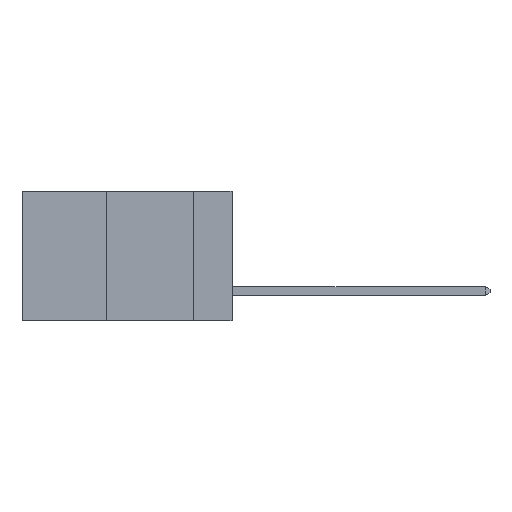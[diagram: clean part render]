
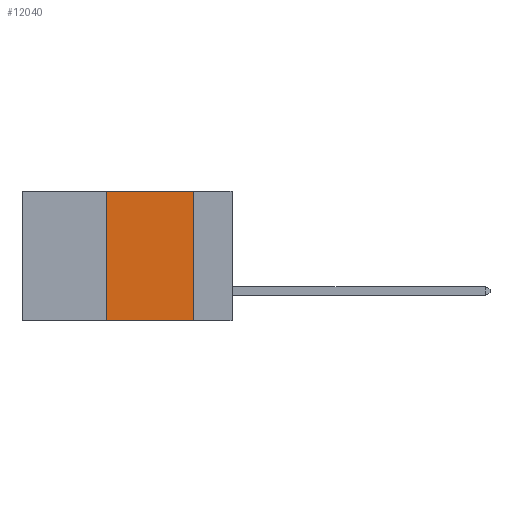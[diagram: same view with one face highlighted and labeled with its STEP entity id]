
A CAD part, left-side view. The second image highlights one B-rep face of the part: STEP entity #12040.
In plain terms, the highlighted planar face has unit normal (-1, 0, 0).
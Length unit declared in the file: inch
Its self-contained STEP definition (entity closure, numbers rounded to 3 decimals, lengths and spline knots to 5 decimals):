
#371 = EDGE_CURVE ( 'NONE', #9237, #3253, #4774, .T. ) ;
#499 = DIRECTION ( 'NONE',  ( 0., 0., 1. ) ) ;
#1607 = ORIENTED_EDGE ( 'NONE', *, *, #371, .F. ) ;
#1988 = ORIENTED_EDGE ( 'NONE', *, *, #7196, .T. ) ;
#2389 = EDGE_LOOP ( 'NONE', ( #4453, #13471, #1607, #1988 ) ) ;
#2433 = DIRECTION ( 'NONE',  ( 0., 0., -1. ) ) ;
#2505 = EDGE_CURVE ( 'NONE', #3253, #5247, #14600, .T. ) ;
#2654 = CARTESIAN_POINT ( 'NONE',  ( 0., 0.6, -0.37 ) ) ;
#2707 = DIRECTION ( 'NONE',  ( 0., -1., 0. ) ) ;
#2745 = CARTESIAN_POINT ( 'NONE',  ( 0., 0.11, 0. ) ) ;
#3253 = VERTEX_POINT ( 'NONE', #8186 ) ;
#3394 = CARTESIAN_POINT ( 'NONE',  ( 0., 0.11, 0. ) ) ;
#3473 = VECTOR ( 'NONE', #5150, 39.37008 ) ;
#4453 = ORIENTED_EDGE ( 'NONE', *, *, #7856, .F. ) ;
#4774 = LINE ( 'NONE', #5841, #7507 ) ;
#4916 = AXIS2_PLACEMENT_3D ( 'NONE', #11189, #9439, #2433 ) ;
#4952 = VECTOR ( 'NONE', #7003, 39.37008 ) ;
#5150 = DIRECTION ( 'NONE',  ( 0., 0., -1. ) ) ;
#5247 = VERTEX_POINT ( 'NONE', #3394 ) ;
#5821 = CARTESIAN_POINT ( 'NONE',  ( 0., 0.6, 0. ) ) ;
#5841 = CARTESIAN_POINT ( 'NONE',  ( 0., 0.36, 0. ) ) ;
#6643 = LINE ( 'NONE', #2745, #3473 ) ;
#7003 = DIRECTION ( 'NONE',  ( 0., -1., 0. ) ) ;
#7159 = PLANE ( 'NONE',  #4916 ) ;
#7196 = EDGE_CURVE ( 'NONE', #9237, #13325, #10532, .T. ) ;
#7507 = VECTOR ( 'NONE', #499, 39.37008 ) ;
#7567 = VECTOR ( 'NONE', #2707, 39.37008 ) ;
#7856 = EDGE_CURVE ( 'NONE', #5247, #13325, #6643, .T. ) ;
#8186 = CARTESIAN_POINT ( 'NONE',  ( 0., 0.36, 0. ) ) ;
#9237 = VERTEX_POINT ( 'NONE', #11352 ) ;
#9407 = CARTESIAN_POINT ( 'NONE',  ( 0., 0.11, -0.37 ) ) ;
#9439 = DIRECTION ( 'NONE',  ( 1., 0., 0. ) ) ;
#10532 = LINE ( 'NONE', #2654, #7567 ) ;
#11189 = CARTESIAN_POINT ( 'NONE',  ( 0., 0.6, 0. ) ) ;
#11352 = CARTESIAN_POINT ( 'NONE',  ( 0., 0.36, -0.37 ) ) ;
#12040 = ADVANCED_FACE ( 'NONE', ( #13808 ), #7159, .F. ) ;
#13325 = VERTEX_POINT ( 'NONE', #9407 ) ;
#13471 = ORIENTED_EDGE ( 'NONE', *, *, #2505, .F. ) ;
#13808 = FACE_OUTER_BOUND ( 'NONE', #2389, .T. ) ;
#14600 = LINE ( 'NONE', #5821, #4952 ) ;
